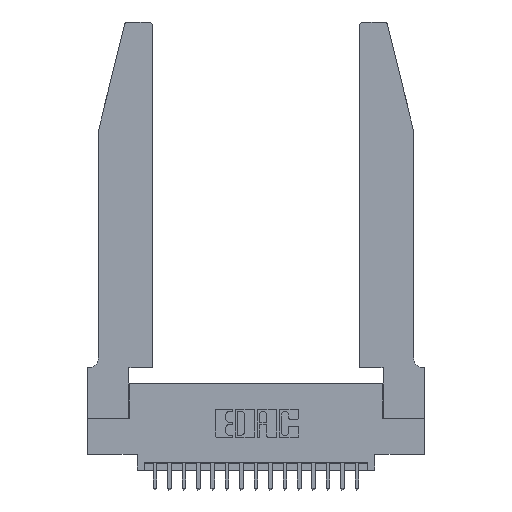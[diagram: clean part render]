
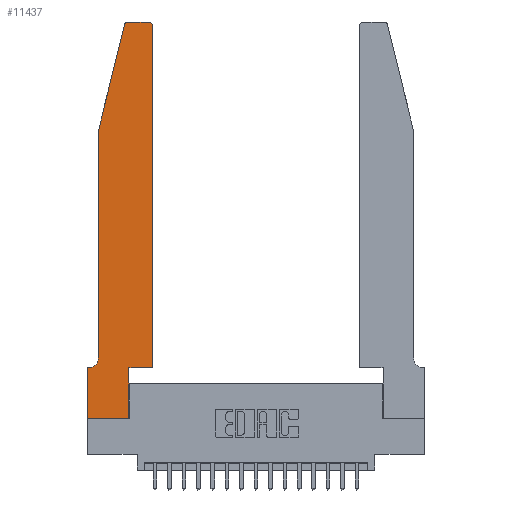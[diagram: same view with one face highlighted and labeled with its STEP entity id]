
A CAD part, top view. The second image highlights one B-rep face of the part: STEP entity #11437.
In plain terms, the highlighted planar face has unit normal (0, 0, 1).
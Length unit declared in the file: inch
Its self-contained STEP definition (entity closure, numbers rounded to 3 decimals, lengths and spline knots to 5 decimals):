
#169 = DIRECTION ( 'NONE',  ( 0., 0., -1. ) ) ;
#206 = CIRCLE ( 'NONE', #16292, 0.03 ) ;
#208 = DIRECTION ( 'NONE',  ( -0.239, -0.971, 0. ) ) ;
#296 = DIRECTION ( 'NONE',  ( 1., 0., 0. ) ) ;
#570 = VECTOR ( 'NONE', #15429, 39.37008 ) ;
#577 = DIRECTION ( 'NONE',  ( 0., 0., 1. ) ) ;
#893 = VERTEX_POINT ( 'NONE', #19162 ) ;
#908 = VERTEX_POINT ( 'NONE', #12793 ) ;
#1177 = CARTESIAN_POINT ( 'NONE',  ( 0.4205, 2.72, 0.37 ) ) ;
#1272 = DIRECTION ( 'NONE',  ( 0., 1., 0. ) ) ;
#1628 = VERTEX_POINT ( 'NONE', #17238 ) ;
#1782 = AXIS2_PLACEMENT_3D ( 'NONE', #19120, #9789, #296 ) ;
#1881 = ORIENTED_EDGE ( 'NONE', *, *, #19805, .T. ) ;
#2041 = LINE ( 'NONE', #5870, #18227 ) ;
#2061 = VECTOR ( 'NONE', #14066, 39.37008 ) ;
#2326 = VERTEX_POINT ( 'NONE', #17493 ) ;
#2474 = EDGE_LOOP ( 'NONE', ( #13842, #10877, #5990, #1881, #8057, #19133, #7931, #16400, #13743, #14110, #10057, #5658 ) ) ;
#2781 = DIRECTION ( 'NONE',  ( 1., 0., 0. ) ) ;
#2877 = EDGE_CURVE ( 'NONE', #6064, #7687, #14625, .T. ) ;
#2943 = EDGE_CURVE ( 'NONE', #13358, #893, #5289, .T. ) ;
#3332 = EDGE_CURVE ( 'NONE', #1628, #908, #2041, .T. ) ;
#3464 = AXIS2_PLACEMENT_3D ( 'NONE', #6884, #577, #11619 ) ;
#3473 = VERTEX_POINT ( 'NONE', #6212 ) ;
#3502 = VECTOR ( 'NONE', #1272, 39.37008 ) ;
#3803 = LINE ( 'NONE', #4454, #570 ) ;
#4454 = CARTESIAN_POINT ( 'NONE',  ( 0.0755, 2., 0.37 ) ) ;
#4722 = LINE ( 'NONE', #15679, #17229 ) ;
#5218 = VECTOR ( 'NONE', #7713, 39.37008 ) ;
#5266 = CARTESIAN_POINT ( 'NONE',  ( 0.0755, 0.42, 0.37 ) ) ;
#5289 = CIRCLE ( 'NONE', #8682, 0.07 ) ;
#5560 = VECTOR ( 'NONE', #208, 39.37008 ) ;
#5658 = ORIENTED_EDGE ( 'NONE', *, *, #9811, .T. ) ;
#5870 = CARTESIAN_POINT ( 'NONE',  ( 0.4505, 0.35, 0.37 ) ) ;
#5990 = ORIENTED_EDGE ( 'NONE', *, *, #19441, .T. ) ;
#6064 = VERTEX_POINT ( 'NONE', #16826 ) ;
#6083 = CARTESIAN_POINT ( 'NONE',  ( 0.2865, 0., 0.37 ) ) ;
#6212 = CARTESIAN_POINT ( 'NONE',  ( 0., 0.35, 0.37 ) ) ;
#6298 = DIRECTION ( 'NONE',  ( 1., 0., 0. ) ) ;
#6884 = CARTESIAN_POINT ( 'NONE',  ( 0., 0.35, 0.37 ) ) ;
#7150 = CARTESIAN_POINT ( 'NONE',  ( 0.0755, 0.35, 0.37 ) ) ;
#7687 = VERTEX_POINT ( 'NONE', #18160 ) ;
#7713 = DIRECTION ( 'NONE',  ( 0., -1., 0. ) ) ;
#7931 = ORIENTED_EDGE ( 'NONE', *, *, #13686, .T. ) ;
#8057 = ORIENTED_EDGE ( 'NONE', *, *, #2943, .T. ) ;
#8682 = AXIS2_PLACEMENT_3D ( 'NONE', #9671, #169, #11244 ) ;
#8918 = EDGE_CURVE ( 'NONE', #19728, #1628, #11390, .T. ) ;
#9393 = EDGE_CURVE ( 'NONE', #18095, #19728, #19625, .T. ) ;
#9671 = CARTESIAN_POINT ( 'NONE',  ( 0.0055, 0.42, 0.37 ) ) ;
#9748 = LINE ( 'NONE', #11217, #5560 ) ;
#9789 = DIRECTION ( 'NONE',  ( 0., 0., 1. ) ) ;
#9811 = EDGE_CURVE ( 'NONE', #908, #6064, #206, .T. ) ;
#10057 = ORIENTED_EDGE ( 'NONE', *, *, #3332, .T. ) ;
#10715 = CARTESIAN_POINT ( 'NONE',  ( 0.2865, 0.35, 0.37 ) ) ;
#10839 = CARTESIAN_POINT ( 'NONE',  ( 0.0755, 2., 0.37 ) ) ;
#10877 = ORIENTED_EDGE ( 'NONE', *, *, #16443, .T. ) ;
#11217 = CARTESIAN_POINT ( 'NONE',  ( 0.0755, 2., 0.37 ) ) ;
#11244 = DIRECTION ( 'NONE',  ( -1., 0., 0. ) ) ;
#11390 = LINE ( 'NONE', #13757, #15050 ) ;
#11437 = ADVANCED_FACE ( 'NONE', ( #15224 ), #19366, .T. ) ;
#11619 = DIRECTION ( 'NONE',  ( 1., 0., 0. ) ) ;
#12210 = DIRECTION ( 'NONE',  ( 0., 0., 1. ) ) ;
#12439 = EDGE_CURVE ( 'NONE', #13245, #18095, #4722, .T. ) ;
#12793 = CARTESIAN_POINT ( 'NONE',  ( 0.4505, 2.72, 0.37 ) ) ;
#13073 = LINE ( 'NONE', #15506, #5218 ) ;
#13245 = VERTEX_POINT ( 'NONE', #14402 ) ;
#13358 = VERTEX_POINT ( 'NONE', #5266 ) ;
#13405 = DIRECTION ( 'NONE',  ( -1., 0., 0. ) ) ;
#13683 = CARTESIAN_POINT ( 'NONE',  ( 0.2865, 0.35, 0.37 ) ) ;
#13686 = EDGE_CURVE ( 'NONE', #3473, #13245, #13073, .T. ) ;
#13743 = ORIENTED_EDGE ( 'NONE', *, *, #9393, .T. ) ;
#13757 = CARTESIAN_POINT ( 'NONE',  ( 0.4505, 0.35, 0.37 ) ) ;
#13842 = ORIENTED_EDGE ( 'NONE', *, *, #2877, .T. ) ;
#14066 = DIRECTION ( 'NONE',  ( -1., 0., 0. ) ) ;
#14110 = ORIENTED_EDGE ( 'NONE', *, *, #8918, .T. ) ;
#14152 = VERTEX_POINT ( 'NONE', #10839 ) ;
#14402 = CARTESIAN_POINT ( 'NONE',  ( 0., 0., 0.37 ) ) ;
#14625 = LINE ( 'NONE', #15617, #2061 ) ;
#15050 = VECTOR ( 'NONE', #16943, 39.37008 ) ;
#15224 = FACE_OUTER_BOUND ( 'NONE', #2474, .T. ) ;
#15429 = DIRECTION ( 'NONE',  ( 0., -1., 0. ) ) ;
#15506 = CARTESIAN_POINT ( 'NONE',  ( 0., 0., 0.37 ) ) ;
#15617 = CARTESIAN_POINT ( 'NONE',  ( 0.2605, 2.75, 0.37 ) ) ;
#15679 = CARTESIAN_POINT ( 'NONE',  ( 0., 0., 0.37 ) ) ;
#16292 = AXIS2_PLACEMENT_3D ( 'NONE', #1177, #12210, #2781 ) ;
#16400 = ORIENTED_EDGE ( 'NONE', *, *, #12439, .T. ) ;
#16443 = EDGE_CURVE ( 'NONE', #7687, #2326, #17087, .T. ) ;
#16826 = CARTESIAN_POINT ( 'NONE',  ( 0.4205, 2.75, 0.37 ) ) ;
#16943 = DIRECTION ( 'NONE',  ( 1., 0., 0. ) ) ;
#17087 = CIRCLE ( 'NONE', #1782, 0.03 ) ;
#17229 = VECTOR ( 'NONE', #6298, 39.37008 ) ;
#17238 = CARTESIAN_POINT ( 'NONE',  ( 0.4505, 0.35, 0.37 ) ) ;
#17493 = CARTESIAN_POINT ( 'NONE',  ( 0.25487, 2.72718, 0.37 ) ) ;
#18095 = VERTEX_POINT ( 'NONE', #6083 ) ;
#18160 = CARTESIAN_POINT ( 'NONE',  ( 0.284, 2.75, 0.37 ) ) ;
#18227 = VECTOR ( 'NONE', #18389, 39.37008 ) ;
#18389 = DIRECTION ( 'NONE',  ( 0., 1., 0. ) ) ;
#19120 = CARTESIAN_POINT ( 'NONE',  ( 0.284, 2.72, 0.37 ) ) ;
#19133 = ORIENTED_EDGE ( 'NONE', *, *, #19613, .T. ) ;
#19162 = CARTESIAN_POINT ( 'NONE',  ( 0.0055, 0.35, 0.37 ) ) ;
#19366 = PLANE ( 'NONE',  #3464 ) ;
#19441 = EDGE_CURVE ( 'NONE', #2326, #14152, #9748, .T. ) ;
#19613 = EDGE_CURVE ( 'NONE', #893, #3473, #19711, .T. ) ;
#19625 = LINE ( 'NONE', #10715, #3502 ) ;
#19711 = LINE ( 'NONE', #7150, #20189 ) ;
#19728 = VERTEX_POINT ( 'NONE', #13683 ) ;
#19805 = EDGE_CURVE ( 'NONE', #14152, #13358, #3803, .T. ) ;
#20189 = VECTOR ( 'NONE', #13405, 39.37008 ) ;
